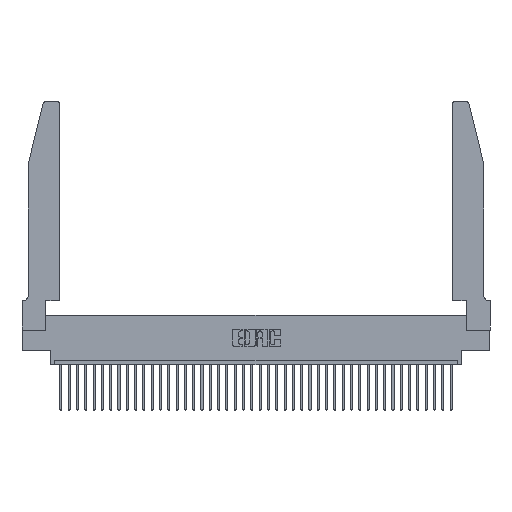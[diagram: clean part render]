
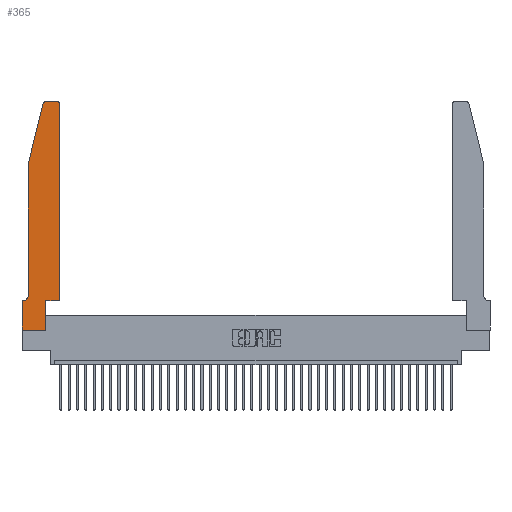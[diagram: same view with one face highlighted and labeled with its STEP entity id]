
A CAD part, top view. The second image highlights one B-rep face of the part: STEP entity #365.
In plain terms, the highlighted planar face has unit normal (0, 0, 1).
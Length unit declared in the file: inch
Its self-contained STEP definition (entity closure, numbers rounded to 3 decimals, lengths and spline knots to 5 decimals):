
#183 = DIRECTION ( 'NONE',  ( 1., 0., 0. ) ) ;
#288 = CARTESIAN_POINT ( 'NONE',  ( 0.0755, 2., 0.37 ) ) ;
#365 = ADVANCED_FACE ( 'NONE', ( #26590 ), #18681, .T. ) ;
#1157 = CARTESIAN_POINT ( 'NONE',  ( 0.25487, 2.72718, 0.37 ) ) ;
#1208 = AXIS2_PLACEMENT_3D ( 'NONE', #17211, #39135, #26686 ) ;
#1900 = CARTESIAN_POINT ( 'NONE',  ( 0.0755, 0.35, 0.37 ) ) ;
#1944 = CARTESIAN_POINT ( 'NONE',  ( 0.2865, 0., 0.37 ) ) ;
#2964 = LINE ( 'NONE', #34783, #9766 ) ;
#3407 = VECTOR ( 'NONE', #6050, 39.37008 ) ;
#3647 = DIRECTION ( 'NONE',  ( -1., 0., 0. ) ) ;
#4121 = VECTOR ( 'NONE', #23070, 39.37008 ) ;
#4310 = ORIENTED_EDGE ( 'NONE', *, *, #13535, .T. ) ;
#4383 = CARTESIAN_POINT ( 'NONE',  ( 0.2865, 0.35, 0.37 ) ) ;
#4617 = CARTESIAN_POINT ( 'NONE',  ( 0., 0., 0.37 ) ) ;
#4652 = VERTEX_POINT ( 'NONE', #1944 ) ;
#5832 = LINE ( 'NONE', #29297, #30700 ) ;
#5864 = LINE ( 'NONE', #33817, #3407 ) ;
#6050 = DIRECTION ( 'NONE',  ( 0., -1., 0. ) ) ;
#6223 = DIRECTION ( 'NONE',  ( 0., 0., 1. ) ) ;
#6290 = EDGE_CURVE ( 'NONE', #17828, #20835, #12420, .T. ) ;
#6492 = DIRECTION ( 'NONE',  ( -0.239, -0.971, 0. ) ) ;
#6684 = ORIENTED_EDGE ( 'NONE', *, *, #16502, .T. ) ;
#7421 = CARTESIAN_POINT ( 'NONE',  ( 0.4505, 0.35, 0.37 ) ) ;
#7734 = ORIENTED_EDGE ( 'NONE', *, *, #24920, .T. ) ;
#7838 = VECTOR ( 'NONE', #23015, 39.37008 ) ;
#8388 = LINE ( 'NONE', #1900, #19535 ) ;
#8775 = EDGE_CURVE ( 'NONE', #4652, #17828, #14191, .T. ) ;
#8853 = EDGE_CURVE ( 'NONE', #20835, #40137, #5832, .T. ) ;
#8926 = DIRECTION ( 'NONE',  ( 1., 0., 0. ) ) ;
#9557 = CARTESIAN_POINT ( 'NONE',  ( 0.0755, 0.42, 0.37 ) ) ;
#9766 = VECTOR ( 'NONE', #31676, 39.37008 ) ;
#9825 = ORIENTED_EDGE ( 'NONE', *, *, #35975, .T. ) ;
#9974 = DIRECTION ( 'NONE',  ( 0., 0., 1. ) ) ;
#10679 = DIRECTION ( 'NONE',  ( 0., 1., 0. ) ) ;
#10791 = CARTESIAN_POINT ( 'NONE',  ( 0., 0., 0.37 ) ) ;
#11566 = LINE ( 'NONE', #4617, #29550 ) ;
#12350 = LINE ( 'NONE', #10791, #23536 ) ;
#12420 = LINE ( 'NONE', #7421, #4121 ) ;
#12751 = ORIENTED_EDGE ( 'NONE', *, *, #32810, .T. ) ;
#13535 = EDGE_CURVE ( 'NONE', #34615, #38878, #2964, .T. ) ;
#14191 = LINE ( 'NONE', #4383, #7838 ) ;
#15053 = CARTESIAN_POINT ( 'NONE',  ( 0.284, 2.75, 0.37 ) ) ;
#15678 = CARTESIAN_POINT ( 'NONE',  ( 0.4205, 2.72, 0.37 ) ) ;
#16025 = ORIENTED_EDGE ( 'NONE', *, *, #28671, .T. ) ;
#16369 = ORIENTED_EDGE ( 'NONE', *, *, #8853, .T. ) ;
#16502 = EDGE_CURVE ( 'NONE', #38755, #4652, #11566, .T. ) ;
#16856 = ORIENTED_EDGE ( 'NONE', *, *, #36368, .T. ) ;
#17211 = CARTESIAN_POINT ( 'NONE',  ( 0.284, 2.72, 0.37 ) ) ;
#17221 = VERTEX_POINT ( 'NONE', #19743 ) ;
#17485 = CIRCLE ( 'NONE', #34100, 0.03 ) ;
#17828 = VERTEX_POINT ( 'NONE', #18330 ) ;
#17883 = VERTEX_POINT ( 'NONE', #1157 ) ;
#18330 = CARTESIAN_POINT ( 'NONE',  ( 0.2865, 0.35, 0.37 ) ) ;
#18681 = PLANE ( 'NONE',  #33111 ) ;
#19021 = ORIENTED_EDGE ( 'NONE', *, *, #33867, .T. ) ;
#19535 = VECTOR ( 'NONE', #32731, 39.37008 ) ;
#19720 = VECTOR ( 'NONE', #6492, 39.37008 ) ;
#19743 = CARTESIAN_POINT ( 'NONE',  ( 0.0755, 2., 0.37 ) ) ;
#20115 = VERTEX_POINT ( 'NONE', #25491 ) ;
#20500 = VERTEX_POINT ( 'NONE', #9557 ) ;
#20835 = VERTEX_POINT ( 'NONE', #30449 ) ;
#21635 = EDGE_CURVE ( 'NONE', #20500, #20115, #32750, .T. ) ;
#23015 = DIRECTION ( 'NONE',  ( 0., 1., 0. ) ) ;
#23070 = DIRECTION ( 'NONE',  ( 1., 0., 0. ) ) ;
#23536 = VECTOR ( 'NONE', #35877, 39.37008 ) ;
#24538 = CIRCLE ( 'NONE', #1208, 0.03 ) ;
#24920 = EDGE_CURVE ( 'NONE', #20115, #30379, #8388, .T. ) ;
#25491 = CARTESIAN_POINT ( 'NONE',  ( 0.0055, 0.35, 0.37 ) ) ;
#26590 = FACE_OUTER_BOUND ( 'NONE', #33418, .T. ) ;
#26686 = DIRECTION ( 'NONE',  ( 1., 0., 0. ) ) ;
#26963 = DIRECTION ( 'NONE',  ( 1., 0., 0. ) ) ;
#27438 = ORIENTED_EDGE ( 'NONE', *, *, #8775, .T. ) ;
#27531 = CARTESIAN_POINT ( 'NONE',  ( 0., 0.35, 0.37 ) ) ;
#28439 = DIRECTION ( 'NONE',  ( 0., 0., -1. ) ) ;
#28636 = AXIS2_PLACEMENT_3D ( 'NONE', #37586, #28439, #3647 ) ;
#28671 = EDGE_CURVE ( 'NONE', #40137, #34615, #17485, .T. ) ;
#29297 = CARTESIAN_POINT ( 'NONE',  ( 0.4505, 0.35, 0.37 ) ) ;
#29550 = VECTOR ( 'NONE', #26963, 39.37008 ) ;
#29845 = ORIENTED_EDGE ( 'NONE', *, *, #21635, .T. ) ;
#30379 = VERTEX_POINT ( 'NONE', #32266 ) ;
#30449 = CARTESIAN_POINT ( 'NONE',  ( 0.4505, 0.35, 0.37 ) ) ;
#30700 = VECTOR ( 'NONE', #10679, 39.37008 ) ;
#31181 = CARTESIAN_POINT ( 'NONE',  ( 0.4205, 2.75, 0.37 ) ) ;
#31676 = DIRECTION ( 'NONE',  ( -1., 0., 0. ) ) ;
#31857 = ORIENTED_EDGE ( 'NONE', *, *, #6290, .T. ) ;
#32266 = CARTESIAN_POINT ( 'NONE',  ( 0., 0.35, 0.37 ) ) ;
#32727 = CARTESIAN_POINT ( 'NONE',  ( 0., 0., 0.37 ) ) ;
#32731 = DIRECTION ( 'NONE',  ( -1., 0., 0. ) ) ;
#32750 = CIRCLE ( 'NONE', #28636, 0.07 ) ;
#32810 = EDGE_CURVE ( 'NONE', #30379, #38755, #12350, .T. ) ;
#33111 = AXIS2_PLACEMENT_3D ( 'NONE', #27531, #6223, #8926 ) ;
#33418 = EDGE_LOOP ( 'NONE', ( #4310, #16856, #9825, #19021, #29845, #7734, #12751, #6684, #27438, #31857, #16369, #16025 ) ) ;
#33817 = CARTESIAN_POINT ( 'NONE',  ( 0.0755, 2., 0.37 ) ) ;
#33867 = EDGE_CURVE ( 'NONE', #17221, #20500, #5864, .T. ) ;
#34100 = AXIS2_PLACEMENT_3D ( 'NONE', #15678, #9974, #183 ) ;
#34615 = VERTEX_POINT ( 'NONE', #31181 ) ;
#34783 = CARTESIAN_POINT ( 'NONE',  ( 0.2605, 2.75, 0.37 ) ) ;
#35877 = DIRECTION ( 'NONE',  ( 0., -1., 0. ) ) ;
#35975 = EDGE_CURVE ( 'NONE', #17883, #17221, #36233, .T. ) ;
#36233 = LINE ( 'NONE', #288, #19720 ) ;
#36368 = EDGE_CURVE ( 'NONE', #38878, #17883, #24538, .T. ) ;
#37023 = CARTESIAN_POINT ( 'NONE',  ( 0.4505, 2.72, 0.37 ) ) ;
#37586 = CARTESIAN_POINT ( 'NONE',  ( 0.0055, 0.42, 0.37 ) ) ;
#38755 = VERTEX_POINT ( 'NONE', #32727 ) ;
#38878 = VERTEX_POINT ( 'NONE', #15053 ) ;
#39135 = DIRECTION ( 'NONE',  ( 0., 0., 1. ) ) ;
#40137 = VERTEX_POINT ( 'NONE', #37023 ) ;
